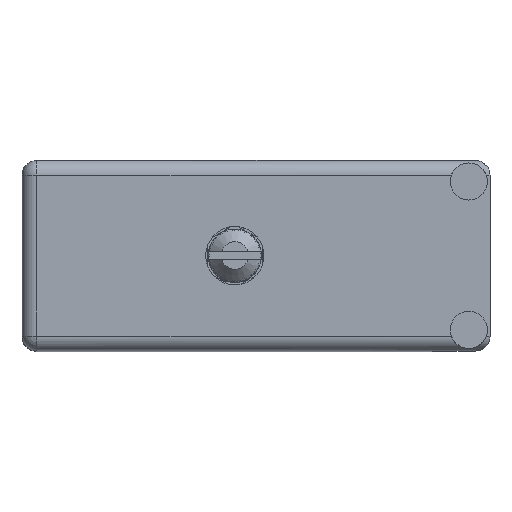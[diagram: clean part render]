
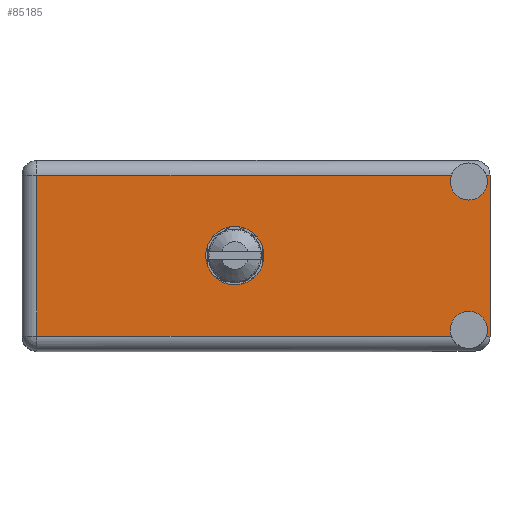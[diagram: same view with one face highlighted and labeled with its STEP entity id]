
A CAD part, top view. The second image highlights one B-rep face of the part: STEP entity #85185.
In plain terms, the highlighted face is planar.
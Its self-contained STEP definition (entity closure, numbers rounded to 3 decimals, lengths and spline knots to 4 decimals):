
#1212 = FACE_BOUND ( 'NONE', #17406, .T. ) ;
#2571 = CIRCLE ( 'NONE', #98256, 0.1375 ) ;
#3739 = CARTESIAN_POINT ( 'NONE',  ( 1.004, 1.566, -0.312 ) ) ;
#4078 = VERTEX_POINT ( 'NONE', #85779 ) ;
#5100 = LINE ( 'NONE', #7892, #85049 ) ;
#5691 = CARTESIAN_POINT ( 'NONE',  ( 2.0256, 1.566, -0.829 ) ) ;
#7470 = VECTOR ( 'NONE', #60868, 39.3701 ) ;
#7892 = CARTESIAN_POINT ( 'NONE',  ( 2.208, 1.566, 0. ) ) ;
#9008 = EDGE_CURVE ( 'NONE', #13012, #30189, #95760, .T. ) ;
#9727 = DIRECTION ( 'NONE',  ( 0., 1., 0. ) ) ;
#10885 = LINE ( 'NONE', #17884, #63670 ) ;
#12514 = ORIENTED_EDGE ( 'NONE', *, *, #9008, .T. ) ;
#12841 = EDGE_CURVE ( 'NONE', #22843, #4078, #22257, .T. ) ;
#13012 = VERTEX_POINT ( 'NONE', #5691 ) ;
#13188 = EDGE_CURVE ( 'NONE', #30189, #80371, #46803, .T. ) ;
#14675 = ORIENTED_EDGE ( 'NONE', *, *, #74252, .T. ) ;
#15659 = EDGE_CURVE ( 'NONE', #87720, #41053, #59336, .T. ) ;
#17406 = EDGE_LOOP ( 'NONE', ( #91157, #104976 ) ) ;
#17884 = CARTESIAN_POINT ( 'NONE',  ( 0., 1.566, -0.829 ) ) ;
#19197 = DIRECTION ( 'NONE',  ( 0., 0., 1. ) ) ;
#20111 = EDGE_CURVE ( 'NONE', #80371, #58981, #50982, .T. ) ;
#20790 = DIRECTION ( 'NONE',  ( -1., 0., 0. ) ) ;
#22100 = AXIS2_PLACEMENT_3D ( 'NONE', #92297, #42539, #84072 ) ;
#22257 = CIRCLE ( 'NONE', #93062, 0.1375 ) ;
#22505 = CIRCLE ( 'NONE', #22100, 0.0875 ) ;
#22843 = VERTEX_POINT ( 'NONE', #3739 ) ;
#22946 = ORIENTED_EDGE ( 'NONE', *, *, #35024, .F. ) ;
#24914 = CARTESIAN_POINT ( 'NONE',  ( 2.0256, 1.566, -0.07 ) ) ;
#25505 = DIRECTION ( 'NONE',  ( 0., 0., 1. ) ) ;
#25753 = ORIENTED_EDGE ( 'NONE', *, *, #20111, .T. ) ;
#26704 = PLANE ( 'NONE',  #27735 ) ;
#27735 = AXIS2_PLACEMENT_3D ( 'NONE', #67737, #93333, #84419 ) ;
#30189 = VERTEX_POINT ( 'NONE', #93301 ) ;
#31288 = AXIS2_PLACEMENT_3D ( 'NONE', #95618, #54526, #63191 ) ;
#31690 = CARTESIAN_POINT ( 'NONE',  ( 2.108, 1.566, -0.712 ) ) ;
#31901 = DIRECTION ( 'NONE',  ( 0., 1., 0. ) ) ;
#33005 = VERTEX_POINT ( 'NONE', #54055 ) ;
#33390 = DIRECTION ( 'NONE',  ( 0., 1., 0. ) ) ;
#35024 = EDGE_CURVE ( 'NONE', #97799, #33005, #86462, .T. ) ;
#39373 = VECTOR ( 'NONE', #40279, 39.3701 ) ;
#40172 = DIRECTION ( 'NONE',  ( 0., 0., 1. ) ) ;
#40279 = DIRECTION ( 'NONE',  ( 1., 0., 0. ) ) ;
#41053 = VERTEX_POINT ( 'NONE', #53036 ) ;
#42247 = AXIS2_PLACEMENT_3D ( 'NONE', #106160, #31901, #40172 ) ;
#42539 = DIRECTION ( 'NONE',  ( 0., 1., 0. ) ) ;
#42764 = CARTESIAN_POINT ( 'NONE',  ( 1.004, 1.566, -0.4495 ) ) ;
#44088 = CARTESIAN_POINT ( 'NONE',  ( 2.208, 1.566, -0.829 ) ) ;
#44625 = EDGE_CURVE ( 'NONE', #41053, #58981, #98164, .T. ) ;
#45287 = CARTESIAN_POINT ( 'NONE',  ( 2.208, 1.566, -0.07 ) ) ;
#45367 = CARTESIAN_POINT ( 'NONE',  ( 2.1904, 1.566, -0.07 ) ) ;
#45639 = VERTEX_POINT ( 'NONE', #44088 ) ;
#46803 = LINE ( 'NONE', #50618, #102163 ) ;
#50618 = CARTESIAN_POINT ( 'NONE',  ( 0.07, 1.566, -0.899 ) ) ;
#50982 = LINE ( 'NONE', #104826, #39373 ) ;
#51210 = DIRECTION ( 'NONE',  ( 0., 1., 0. ) ) ;
#51329 = DIRECTION ( 'NONE',  ( -1., 0., 0. ) ) ;
#52712 = EDGE_CURVE ( 'NONE', #45639, #33005, #10885, .T. ) ;
#53036 = CARTESIAN_POINT ( 'NONE',  ( 2.108, 1.566, -0.187 ) ) ;
#53671 = ORIENTED_EDGE ( 'NONE', *, *, #52712, .T. ) ;
#54055 = CARTESIAN_POINT ( 'NONE',  ( 2.1904, 1.566, -0.829 ) ) ;
#54526 = DIRECTION ( 'NONE',  ( 0., 1., 0. ) ) ;
#57284 = EDGE_CURVE ( 'NONE', #4078, #22843, #2571, .T. ) ;
#58981 = VERTEX_POINT ( 'NONE', #24914 ) ;
#59132 = FACE_OUTER_BOUND ( 'NONE', #60595, .T. ) ;
#59336 = CIRCLE ( 'NONE', #42247, 0.0875 ) ;
#60595 = EDGE_LOOP ( 'NONE', ( #25753, #68534, #65760, #14675, #75339, #53671, #22946, #80675, #12514, #92087 ) ) ;
#60868 = DIRECTION ( 'NONE',  ( 1., 0., 0. ) ) ;
#62860 = CARTESIAN_POINT ( 'NONE',  ( 0., 1.566, -0.829 ) ) ;
#63191 = DIRECTION ( 'NONE',  ( 0., 0., 1. ) ) ;
#63670 = VECTOR ( 'NONE', #51329, 39.3701 ) ;
#65760 = ORIENTED_EDGE ( 'NONE', *, *, #15659, .F. ) ;
#66192 = CARTESIAN_POINT ( 'NONE',  ( 1.004, 1.566, -0.4495 ) ) ;
#67737 = CARTESIAN_POINT ( 'NONE',  ( 0., 1.566, -0.899 ) ) ;
#67871 = AXIS2_PLACEMENT_3D ( 'NONE', #68470, #51210, #19197 ) ;
#68470 = CARTESIAN_POINT ( 'NONE',  ( 2.108, 1.566, -0.0995 ) ) ;
#68534 = ORIENTED_EDGE ( 'NONE', *, *, #44625, .F. ) ;
#69896 = VERTEX_POINT ( 'NONE', #45287 ) ;
#74252 = EDGE_CURVE ( 'NONE', #87720, #69896, #89933, .T. ) ;
#75210 = VECTOR ( 'NONE', #20790, 39.3701 ) ;
#75339 = ORIENTED_EDGE ( 'NONE', *, *, #100716, .F. ) ;
#80371 = VERTEX_POINT ( 'NONE', #106857 ) ;
#80675 = ORIENTED_EDGE ( 'NONE', *, *, #90341, .F. ) ;
#84072 = DIRECTION ( 'NONE',  ( 0., 0., 1. ) ) ;
#84419 = DIRECTION ( 'NONE',  ( 0., 0., 1. ) ) ;
#85049 = VECTOR ( 'NONE', #90357, 39.3701 ) ;
#85185 = ADVANCED_FACE ( 'NONE', ( #1212, #59132 ), #26704, .T. ) ;
#85779 = CARTESIAN_POINT ( 'NONE',  ( 1.004, 1.566, -0.587 ) ) ;
#86462 = CIRCLE ( 'NONE', #31288, 0.0875 ) ;
#87720 = VERTEX_POINT ( 'NONE', #45367 ) ;
#89933 = LINE ( 'NONE', #94013, #7470 ) ;
#90034 = DIRECTION ( 'NONE',  ( 0., 0., 1. ) ) ;
#90341 = EDGE_CURVE ( 'NONE', #13012, #97799, #22505, .T. ) ;
#90357 = DIRECTION ( 'NONE',  ( 0., 0., 1. ) ) ;
#91157 = ORIENTED_EDGE ( 'NONE', *, *, #12841, .F. ) ;
#92087 = ORIENTED_EDGE ( 'NONE', *, *, #13188, .T. ) ;
#92297 = CARTESIAN_POINT ( 'NONE',  ( 2.108, 1.566, -0.7995 ) ) ;
#93062 = AXIS2_PLACEMENT_3D ( 'NONE', #42764, #9727, #25505 ) ;
#93301 = CARTESIAN_POINT ( 'NONE',  ( 0.07, 1.566, -0.829 ) ) ;
#93333 = DIRECTION ( 'NONE',  ( 0., 1., 0. ) ) ;
#94013 = CARTESIAN_POINT ( 'NONE',  ( 2.208, 1.566, -0.07 ) ) ;
#95618 = CARTESIAN_POINT ( 'NONE',  ( 2.108, 1.566, -0.7995 ) ) ;
#95760 = LINE ( 'NONE', #62860, #75210 ) ;
#97799 = VERTEX_POINT ( 'NONE', #31690 ) ;
#98164 = CIRCLE ( 'NONE', #67871, 0.0875 ) ;
#98256 = AXIS2_PLACEMENT_3D ( 'NONE', #66192, #33390, #90034 ) ;
#100716 = EDGE_CURVE ( 'NONE', #45639, #69896, #5100, .T. ) ;
#101438 = DIRECTION ( 'NONE',  ( 0., 0., 1. ) ) ;
#102163 = VECTOR ( 'NONE', #101438, 39.3701 ) ;
#104826 = CARTESIAN_POINT ( 'NONE',  ( 2.208, 1.566, -0.07 ) ) ;
#104976 = ORIENTED_EDGE ( 'NONE', *, *, #57284, .F. ) ;
#106160 = CARTESIAN_POINT ( 'NONE',  ( 2.108, 1.566, -0.0995 ) ) ;
#106857 = CARTESIAN_POINT ( 'NONE',  ( 0.07, 1.566, -0.07 ) ) ;
